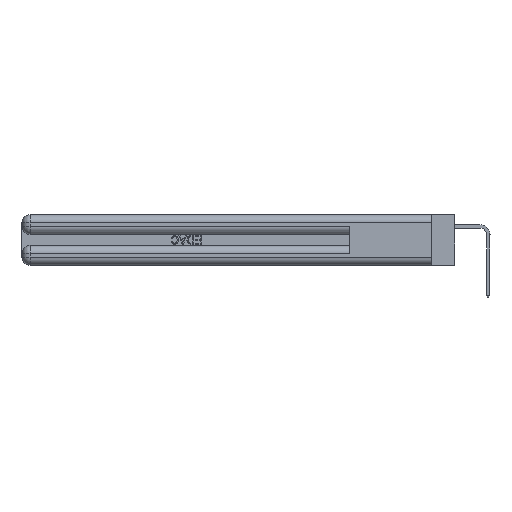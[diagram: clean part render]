
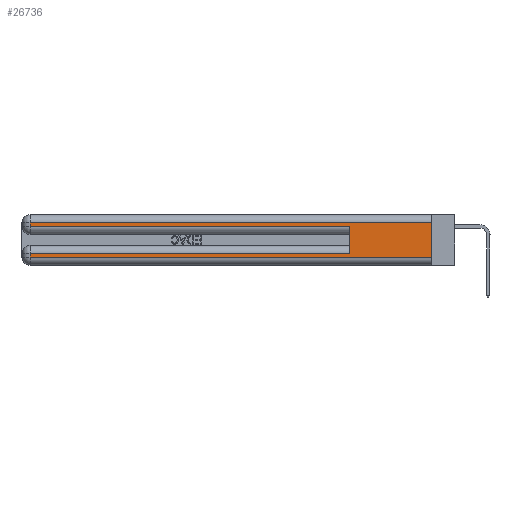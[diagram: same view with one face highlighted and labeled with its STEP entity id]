
A CAD part, left-side view. The second image highlights one B-rep face of the part: STEP entity #26736.
In plain terms, the highlighted planar face has unit normal (-1, 0, 0).
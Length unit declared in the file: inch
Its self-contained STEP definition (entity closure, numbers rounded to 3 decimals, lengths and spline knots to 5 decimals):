
#193 = LINE ( 'NONE', #24150, #42361 ) ;
#380 = DIRECTION ( 'NONE',  ( 0., 1., 0. ) ) ;
#1949 = DIRECTION ( 'NONE',  ( 0., -1., 0. ) ) ;
#2394 = CARTESIAN_POINT ( 'NONE',  ( 0., 0., 0.06 ) ) ;
#2564 = CARTESIAN_POINT ( 'NONE',  ( 0., 2.94, 0.37 ) ) ;
#2616 = VECTOR ( 'NONE', #32013, 39.37008 ) ;
#2700 = ORIENTED_EDGE ( 'NONE', *, *, #2869, .T. ) ;
#2869 = EDGE_CURVE ( 'NONE', #39917, #38414, #193, .T. ) ;
#3031 = VECTOR ( 'NONE', #25036, 39.37008 ) ;
#3877 = LINE ( 'NONE', #39929, #2616 ) ;
#4206 = LINE ( 'NONE', #40666, #14831 ) ;
#4935 = ORIENTED_EDGE ( 'NONE', *, *, #27265, .T. ) ;
#5314 = VERTEX_POINT ( 'NONE', #26991 ) ;
#5903 = PLANE ( 'NONE',  #18065 ) ;
#5996 = CARTESIAN_POINT ( 'NONE',  ( 0., 0., 0.285 ) ) ;
#9226 = LINE ( 'NONE', #2564, #29023 ) ;
#9746 = CARTESIAN_POINT ( 'NONE',  ( 0., 0.6, 0.085 ) ) ;
#9921 = DIRECTION ( 'NONE',  ( 0., 0., -1. ) ) ;
#12165 = EDGE_CURVE ( 'NONE', #26722, #26069, #28595, .T. ) ;
#13047 = DIRECTION ( 'NONE',  ( 0., -1., 0. ) ) ;
#13187 = CARTESIAN_POINT ( 'NONE',  ( 0., 2.94, 0.37 ) ) ;
#13294 = VERTEX_POINT ( 'NONE', #18044 ) ;
#13761 = CARTESIAN_POINT ( 'NONE',  ( 0., 0., 0.37 ) ) ;
#14831 = VECTOR ( 'NONE', #13047, 39.37008 ) ;
#15495 = VERTEX_POINT ( 'NONE', #42148 ) ;
#15518 = LINE ( 'NONE', #44477, #34053 ) ;
#18044 = CARTESIAN_POINT ( 'NONE',  ( 0., 2.94, 0.06 ) ) ;
#18065 = AXIS2_PLACEMENT_3D ( 'NONE', #13761, #33595, #9921 ) ;
#23193 = VECTOR ( 'NONE', #1949, 39.37008 ) ;
#24122 = LINE ( 'NONE', #13187, #3031 ) ;
#24150 = CARTESIAN_POINT ( 'NONE',  ( 0., 0., 0.31 ) ) ;
#25036 = DIRECTION ( 'NONE',  ( 0., 0., -1. ) ) ;
#25234 = EDGE_CURVE ( 'NONE', #39917, #45540, #3877, .T. ) ;
#26069 = VERTEX_POINT ( 'NONE', #33658 ) ;
#26722 = VERTEX_POINT ( 'NONE', #9746 ) ;
#26736 = ADVANCED_FACE ( 'NONE', ( #37159 ), #5903, .F. ) ;
#26991 = CARTESIAN_POINT ( 'NONE',  ( 0., 2.94, 0.285 ) ) ;
#27265 = EDGE_CURVE ( 'NONE', #38414, #5314, #24122, .T. ) ;
#27488 = CARTESIAN_POINT ( 'NONE',  ( 0., 0., 0.085 ) ) ;
#28595 = LINE ( 'NONE', #27488, #48297 ) ;
#29023 = VECTOR ( 'NONE', #50103, 39.37008 ) ;
#30239 = ORIENTED_EDGE ( 'NONE', *, *, #42502, .T. ) ;
#31487 = DIRECTION ( 'NONE',  ( 0., 1., 0. ) ) ;
#31914 = EDGE_CURVE ( 'NONE', #26722, #15495, #15518, .T. ) ;
#32013 = DIRECTION ( 'NONE',  ( 0., 0., -1. ) ) ;
#33595 = DIRECTION ( 'NONE',  ( 1., 0., 0. ) ) ;
#33658 = CARTESIAN_POINT ( 'NONE',  ( 0., 2.94, 0.085 ) ) ;
#34053 = VECTOR ( 'NONE', #48418, 39.37008 ) ;
#36093 = CARTESIAN_POINT ( 'NONE',  ( 0., 2.94, 0.31 ) ) ;
#37159 = FACE_OUTER_BOUND ( 'NONE', #38388, .T. ) ;
#38388 = EDGE_LOOP ( 'NONE', ( #40872, #2700, #4935, #41602, #40214, #45694, #45781, #30239 ) ) ;
#38414 = VERTEX_POINT ( 'NONE', #36093 ) ;
#39917 = VERTEX_POINT ( 'NONE', #47314 ) ;
#39929 = CARTESIAN_POINT ( 'NONE',  ( 0., 0., 0.37 ) ) ;
#40214 = ORIENTED_EDGE ( 'NONE', *, *, #31914, .F. ) ;
#40275 = EDGE_CURVE ( 'NONE', #5314, #15495, #44190, .T. ) ;
#40666 = CARTESIAN_POINT ( 'NONE',  ( 0., 0., 0.06 ) ) ;
#40872 = ORIENTED_EDGE ( 'NONE', *, *, #25234, .F. ) ;
#41602 = ORIENTED_EDGE ( 'NONE', *, *, #40275, .T. ) ;
#42148 = CARTESIAN_POINT ( 'NONE',  ( 0., 0.6, 0.285 ) ) ;
#42361 = VECTOR ( 'NONE', #380, 39.37008 ) ;
#42502 = EDGE_CURVE ( 'NONE', #13294, #45540, #4206, .T. ) ;
#44190 = LINE ( 'NONE', #5996, #23193 ) ;
#44477 = CARTESIAN_POINT ( 'NONE',  ( 0., 0.6, 0.145 ) ) ;
#45540 = VERTEX_POINT ( 'NONE', #2394 ) ;
#45694 = ORIENTED_EDGE ( 'NONE', *, *, #12165, .T. ) ;
#45781 = ORIENTED_EDGE ( 'NONE', *, *, #48948, .T. ) ;
#47314 = CARTESIAN_POINT ( 'NONE',  ( 0., 0., 0.31 ) ) ;
#48297 = VECTOR ( 'NONE', #31487, 39.37008 ) ;
#48418 = DIRECTION ( 'NONE',  ( 0., 0., 1. ) ) ;
#48948 = EDGE_CURVE ( 'NONE', #26069, #13294, #9226, .T. ) ;
#50103 = DIRECTION ( 'NONE',  ( 0., 0., -1. ) ) ;
